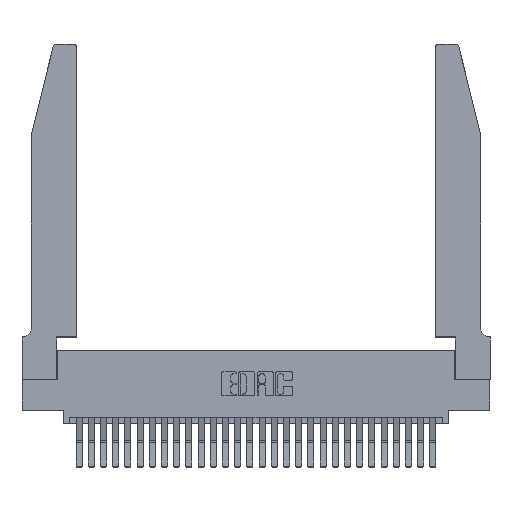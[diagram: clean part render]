
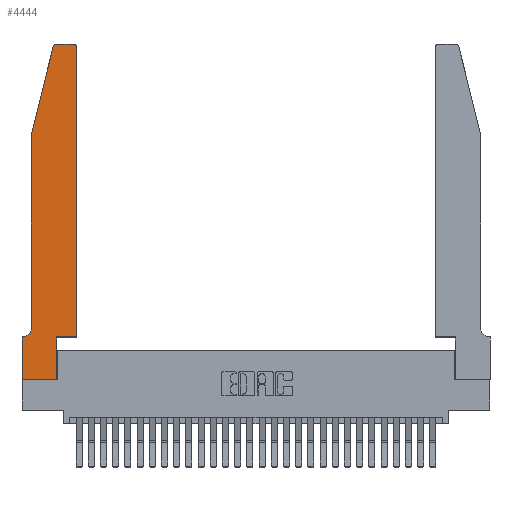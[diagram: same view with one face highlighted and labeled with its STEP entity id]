
A CAD part, top view. The second image highlights one B-rep face of the part: STEP entity #4444.
In plain terms, the highlighted planar face has unit normal (0, 0, 1).
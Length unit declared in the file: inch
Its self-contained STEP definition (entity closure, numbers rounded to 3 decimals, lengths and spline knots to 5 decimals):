
#630 = VERTEX_POINT ( 'NONE', #4789 ) ;
#1680 = EDGE_CURVE ( 'NONE', #17974, #5420, #11307, .T. ) ;
#1875 = CARTESIAN_POINT ( 'NONE',  ( 0.4505, 0.35, 0.37 ) ) ;
#2079 = ORIENTED_EDGE ( 'NONE', *, *, #20560, .T. ) ;
#2189 = CARTESIAN_POINT ( 'NONE',  ( 0., 0.35, 0.37 ) ) ;
#2763 = ORIENTED_EDGE ( 'NONE', *, *, #29758, .T. ) ;
#2849 = DIRECTION ( 'NONE',  ( 0., 1., 0. ) ) ;
#2999 = DIRECTION ( 'NONE',  ( -1., 0., 0. ) ) ;
#3475 = LINE ( 'NONE', #23377, #11528 ) ;
#3617 = CARTESIAN_POINT ( 'NONE',  ( 0.284, 2.75, 0.37 ) ) ;
#4241 = LINE ( 'NONE', #13119, #25701 ) ;
#4280 = EDGE_CURVE ( 'NONE', #27092, #7201, #26334, .T. ) ;
#4444 = ADVANCED_FACE ( 'NONE', ( #29940 ), #6167, .T. ) ;
#4713 = DIRECTION ( 'NONE',  ( 0., 1., 0. ) ) ;
#4759 = CARTESIAN_POINT ( 'NONE',  ( 0.25487, 2.72718, 0.37 ) ) ;
#4789 = CARTESIAN_POINT ( 'NONE',  ( 0.2865, 0.35, 0.37 ) ) ;
#5040 = ORIENTED_EDGE ( 'NONE', *, *, #14420, .T. ) ;
#5044 = VECTOR ( 'NONE', #21815, 39.37008 ) ;
#5420 = VERTEX_POINT ( 'NONE', #16016 ) ;
#6167 = PLANE ( 'NONE',  #28242 ) ;
#7201 = VERTEX_POINT ( 'NONE', #4759 ) ;
#7810 = CARTESIAN_POINT ( 'NONE',  ( 0., 0., 0.37 ) ) ;
#7950 = ORIENTED_EDGE ( 'NONE', *, *, #20784, .T. ) ;
#8127 = DIRECTION ( 'NONE',  ( 0., 0., 1. ) ) ;
#8561 = EDGE_CURVE ( 'NONE', #11630, #630, #10849, .T. ) ;
#9375 = DIRECTION ( 'NONE',  ( -0.239, -0.971, 0. ) ) ;
#9515 = ORIENTED_EDGE ( 'NONE', *, *, #8561, .T. ) ;
#9685 = ORIENTED_EDGE ( 'NONE', *, *, #14628, .T. ) ;
#9891 = LINE ( 'NONE', #7810, #12459 ) ;
#10068 = LINE ( 'NONE', #13489, #12270 ) ;
#10117 = EDGE_LOOP ( 'NONE', ( #5040, #25085, #12390, #16502, #2763, #10634, #29888, #9685, #9515, #2079, #7950, #13899 ) ) ;
#10163 = CARTESIAN_POINT ( 'NONE',  ( 0.2865, 0., 0.37 ) ) ;
#10380 = LINE ( 'NONE', #13979, #28149 ) ;
#10493 = DIRECTION ( 'NONE',  ( 1., 0., 0. ) ) ;
#10634 = ORIENTED_EDGE ( 'NONE', *, *, #12982, .T. ) ;
#10849 = LINE ( 'NONE', #19512, #15228 ) ;
#11109 = DIRECTION ( 'NONE',  ( -1., 0., 0. ) ) ;
#11307 = LINE ( 'NONE', #14596, #5044 ) ;
#11528 = VECTOR ( 'NONE', #4713, 39.37008 ) ;
#11630 = VERTEX_POINT ( 'NONE', #10163 ) ;
#12270 = VECTOR ( 'NONE', #13693, 39.37008 ) ;
#12390 = ORIENTED_EDGE ( 'NONE', *, *, #15683, .T. ) ;
#12459 = VECTOR ( 'NONE', #19399, 39.37008 ) ;
#12982 = EDGE_CURVE ( 'NONE', #21734, #22889, #17405, .T. ) ;
#13119 = CARTESIAN_POINT ( 'NONE',  ( 0.4505, 0.35, 0.37 ) ) ;
#13489 = CARTESIAN_POINT ( 'NONE',  ( 0.2605, 2.75, 0.37 ) ) ;
#13610 = CARTESIAN_POINT ( 'NONE',  ( 0.4205, 2.72, 0.37 ) ) ;
#13693 = DIRECTION ( 'NONE',  ( -1., 0., 0. ) ) ;
#13899 = ORIENTED_EDGE ( 'NONE', *, *, #27358, .T. ) ;
#13979 = CARTESIAN_POINT ( 'NONE',  ( 0.0755, 2., 0.37 ) ) ;
#14420 = EDGE_CURVE ( 'NONE', #22617, #27092, #10068, .T. ) ;
#14596 = CARTESIAN_POINT ( 'NONE',  ( 0.0755, 2., 0.37 ) ) ;
#14628 = EDGE_CURVE ( 'NONE', #25950, #11630, #22078, .T. ) ;
#15168 = CARTESIAN_POINT ( 'NONE',  ( 0.4205, 2.75, 0.37 ) ) ;
#15228 = VECTOR ( 'NONE', #2849, 39.37008 ) ;
#15683 = EDGE_CURVE ( 'NONE', #7201, #17974, #10380, .T. ) ;
#16016 = CARTESIAN_POINT ( 'NONE',  ( 0.0755, 0.42, 0.37 ) ) ;
#16139 = CARTESIAN_POINT ( 'NONE',  ( 0.284, 2.72, 0.37 ) ) ;
#16206 = CARTESIAN_POINT ( 'NONE',  ( 0.4505, 2.72, 0.37 ) ) ;
#16502 = ORIENTED_EDGE ( 'NONE', *, *, #1680, .T. ) ;
#16800 = AXIS2_PLACEMENT_3D ( 'NONE', #16139, #18462, #18161 ) ;
#17028 = DIRECTION ( 'NONE',  ( 1., 0., 0. ) ) ;
#17238 = CARTESIAN_POINT ( 'NONE',  ( 0., 0., 0.37 ) ) ;
#17405 = LINE ( 'NONE', #17706, #25072 ) ;
#17616 = CARTESIAN_POINT ( 'NONE',  ( 0.0055, 0.35, 0.37 ) ) ;
#17706 = CARTESIAN_POINT ( 'NONE',  ( 0.0755, 0.35, 0.37 ) ) ;
#17974 = VERTEX_POINT ( 'NONE', #21015 ) ;
#18161 = DIRECTION ( 'NONE',  ( 1., 0., 0. ) ) ;
#18462 = DIRECTION ( 'NONE',  ( 0., 0., 1. ) ) ;
#19399 = DIRECTION ( 'NONE',  ( 0., -1., 0. ) ) ;
#19512 = CARTESIAN_POINT ( 'NONE',  ( 0.2865, 0.35, 0.37 ) ) ;
#20560 = EDGE_CURVE ( 'NONE', #630, #25451, #4241, .T. ) ;
#20628 = AXIS2_PLACEMENT_3D ( 'NONE', #26103, #28823, #2999 ) ;
#20784 = EDGE_CURVE ( 'NONE', #25451, #28098, #3475, .T. ) ;
#20924 = DIRECTION ( 'NONE',  ( 1., 0., 0. ) ) ;
#21015 = CARTESIAN_POINT ( 'NONE',  ( 0.0755, 2., 0.37 ) ) ;
#21327 = CIRCLE ( 'NONE', #20628, 0.07 ) ;
#21381 = AXIS2_PLACEMENT_3D ( 'NONE', #13610, #22985, #20924 ) ;
#21734 = VERTEX_POINT ( 'NONE', #17616 ) ;
#21815 = DIRECTION ( 'NONE',  ( 0., -1., 0. ) ) ;
#22078 = LINE ( 'NONE', #17238, #25704 ) ;
#22617 = VERTEX_POINT ( 'NONE', #15168 ) ;
#22889 = VERTEX_POINT ( 'NONE', #2189 ) ;
#22985 = DIRECTION ( 'NONE',  ( 0., 0., 1. ) ) ;
#23131 = EDGE_CURVE ( 'NONE', #22889, #25950, #9891, .T. ) ;
#23377 = CARTESIAN_POINT ( 'NONE',  ( 0.4505, 0.35, 0.37 ) ) ;
#24726 = DIRECTION ( 'NONE',  ( 1., 0., 0. ) ) ;
#25072 = VECTOR ( 'NONE', #11109, 39.37008 ) ;
#25085 = ORIENTED_EDGE ( 'NONE', *, *, #4280, .T. ) ;
#25451 = VERTEX_POINT ( 'NONE', #1875 ) ;
#25701 = VECTOR ( 'NONE', #24726, 39.37008 ) ;
#25704 = VECTOR ( 'NONE', #17028, 39.37008 ) ;
#25950 = VERTEX_POINT ( 'NONE', #29305 ) ;
#26103 = CARTESIAN_POINT ( 'NONE',  ( 0.0055, 0.42, 0.37 ) ) ;
#26172 = CIRCLE ( 'NONE', #21381, 0.03 ) ;
#26334 = CIRCLE ( 'NONE', #16800, 0.03 ) ;
#27092 = VERTEX_POINT ( 'NONE', #3617 ) ;
#27358 = EDGE_CURVE ( 'NONE', #28098, #22617, #26172, .T. ) ;
#28098 = VERTEX_POINT ( 'NONE', #16206 ) ;
#28149 = VECTOR ( 'NONE', #9375, 39.37008 ) ;
#28242 = AXIS2_PLACEMENT_3D ( 'NONE', #28934, #8127, #10493 ) ;
#28823 = DIRECTION ( 'NONE',  ( 0., 0., -1. ) ) ;
#28934 = CARTESIAN_POINT ( 'NONE',  ( 0., 0.35, 0.37 ) ) ;
#29305 = CARTESIAN_POINT ( 'NONE',  ( 0., 0., 0.37 ) ) ;
#29758 = EDGE_CURVE ( 'NONE', #5420, #21734, #21327, .T. ) ;
#29888 = ORIENTED_EDGE ( 'NONE', *, *, #23131, .T. ) ;
#29940 = FACE_OUTER_BOUND ( 'NONE', #10117, .T. ) ;
